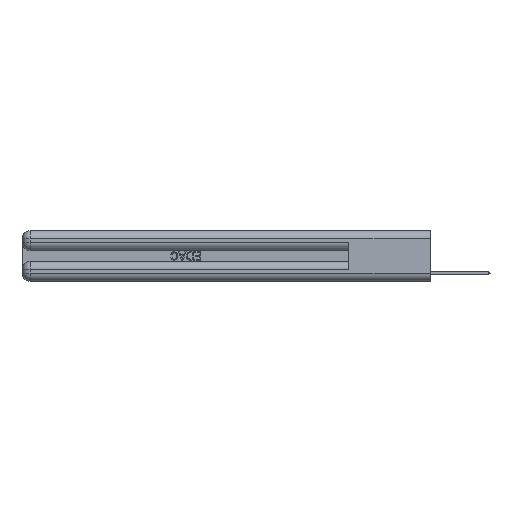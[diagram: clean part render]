
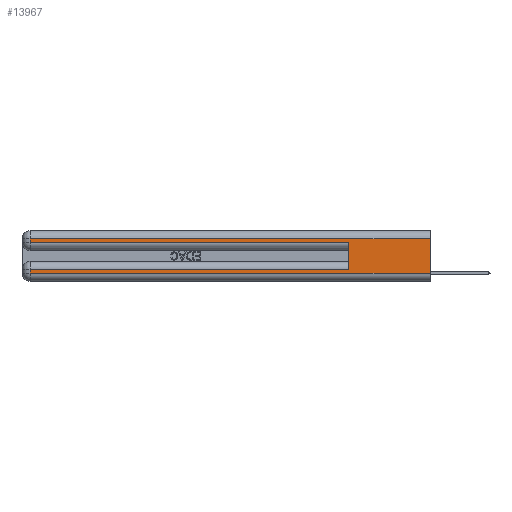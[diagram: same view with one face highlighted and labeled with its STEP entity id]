
A CAD part, left-side view. The second image highlights one B-rep face of the part: STEP entity #13967.
In plain terms, the highlighted planar face has unit normal (-1, 0, 0).
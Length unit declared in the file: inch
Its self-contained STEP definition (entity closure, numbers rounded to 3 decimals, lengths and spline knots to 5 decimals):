
#890 = CARTESIAN_POINT ( 'NONE',  ( 0., 0., 0.37 ) ) ;
#1007 = ORIENTED_EDGE ( 'NONE', *, *, #17822, .T. ) ;
#1080 = ORIENTED_EDGE ( 'NONE', *, *, #3399, .T. ) ;
#1445 = FACE_OUTER_BOUND ( 'NONE', #27630, .T. ) ;
#1595 = LINE ( 'NONE', #23481, #8854 ) ;
#1838 = CARTESIAN_POINT ( 'NONE',  ( 0., 0., 0.06 ) ) ;
#2013 = EDGE_CURVE ( 'NONE', #3633, #29395, #31485, .T. ) ;
#2047 = EDGE_CURVE ( 'NONE', #18196, #31712, #23404, .T. ) ;
#3399 = EDGE_CURVE ( 'NONE', #27878, #25959, #17396, .T. ) ;
#3633 = VERTEX_POINT ( 'NONE', #32773 ) ;
#3682 = VERTEX_POINT ( 'NONE', #33126 ) ;
#4506 = DIRECTION ( 'NONE',  ( 0., 0., -1. ) ) ;
#5807 = CARTESIAN_POINT ( 'NONE',  ( 0., 0., 0.06 ) ) ;
#6829 = ORIENTED_EDGE ( 'NONE', *, *, #7510, .T. ) ;
#7037 = CARTESIAN_POINT ( 'NONE',  ( 0., 2.94, 0.37 ) ) ;
#7241 = VECTOR ( 'NONE', #11696, 39.37008 ) ;
#7389 = CARTESIAN_POINT ( 'NONE',  ( 0., 2.94, 0.37 ) ) ;
#7510 = EDGE_CURVE ( 'NONE', #25959, #31712, #22230, .T. ) ;
#7766 = VECTOR ( 'NONE', #25082, 39.37008 ) ;
#7897 = VECTOR ( 'NONE', #12992, 39.37008 ) ;
#8139 = PLANE ( 'NONE',  #13163 ) ;
#8854 = VECTOR ( 'NONE', #9819, 39.37008 ) ;
#9819 = DIRECTION ( 'NONE',  ( 0., 1., 0. ) ) ;
#11452 = VECTOR ( 'NONE', #25824, 39.37008 ) ;
#11586 = DIRECTION ( 'NONE',  ( 0., 1., 0. ) ) ;
#11696 = DIRECTION ( 'NONE',  ( 0., 0., -1. ) ) ;
#11863 = EDGE_CURVE ( 'NONE', #18196, #24953, #27498, .T. ) ;
#12992 = DIRECTION ( 'NONE',  ( 0., -1., 0. ) ) ;
#13163 = AXIS2_PLACEMENT_3D ( 'NONE', #21433, #29527, #24419 ) ;
#13292 = EDGE_CURVE ( 'NONE', #3682, #29395, #31290, .T. ) ;
#13654 = CARTESIAN_POINT ( 'NONE',  ( 0., 0., 0.31 ) ) ;
#13967 = ADVANCED_FACE ( 'NONE', ( #1445 ), #8139, .F. ) ;
#14440 = VECTOR ( 'NONE', #27520, 39.37008 ) ;
#15915 = CARTESIAN_POINT ( 'NONE',  ( 0., 0., 0.285 ) ) ;
#17396 = LINE ( 'NONE', #7037, #11452 ) ;
#17822 = EDGE_CURVE ( 'NONE', #3633, #27878, #1595, .T. ) ;
#18196 = VERTEX_POINT ( 'NONE', #13654 ) ;
#19053 = CARTESIAN_POINT ( 'NONE',  ( 0., 0.6, 0.145 ) ) ;
#19664 = CARTESIAN_POINT ( 'NONE',  ( 0., 0., 0.31 ) ) ;
#20230 = VECTOR ( 'NONE', #11586, 39.37008 ) ;
#21433 = CARTESIAN_POINT ( 'NONE',  ( 0., 0., 0.37 ) ) ;
#22230 = LINE ( 'NONE', #5807, #7766 ) ;
#22785 = CARTESIAN_POINT ( 'NONE',  ( 0., 2.94, 0.06 ) ) ;
#23404 = LINE ( 'NONE', #890, #7241 ) ;
#23481 = CARTESIAN_POINT ( 'NONE',  ( 0., 0., 0.085 ) ) ;
#23975 = LINE ( 'NONE', #7389, #26538 ) ;
#24419 = DIRECTION ( 'NONE',  ( 0., 0., -1. ) ) ;
#24537 = CARTESIAN_POINT ( 'NONE',  ( 0., 0.6, 0.285 ) ) ;
#24571 = CARTESIAN_POINT ( 'NONE',  ( 0., 2.94, 0.085 ) ) ;
#24953 = VERTEX_POINT ( 'NONE', #30999 ) ;
#24978 = ORIENTED_EDGE ( 'NONE', *, *, #2013, .F. ) ;
#25082 = DIRECTION ( 'NONE',  ( 0., -1., 0. ) ) ;
#25824 = DIRECTION ( 'NONE',  ( 0., 0., -1. ) ) ;
#25959 = VERTEX_POINT ( 'NONE', #22785 ) ;
#26174 = ORIENTED_EDGE ( 'NONE', *, *, #13292, .T. ) ;
#26538 = VECTOR ( 'NONE', #4506, 39.37008 ) ;
#27037 = ORIENTED_EDGE ( 'NONE', *, *, #11863, .T. ) ;
#27457 = ORIENTED_EDGE ( 'NONE', *, *, #2047, .F. ) ;
#27498 = LINE ( 'NONE', #19664, #20230 ) ;
#27520 = DIRECTION ( 'NONE',  ( 0., 0., 1. ) ) ;
#27630 = EDGE_LOOP ( 'NONE', ( #27457, #27037, #33815, #26174, #24978, #1007, #1080, #6829 ) ) ;
#27878 = VERTEX_POINT ( 'NONE', #24571 ) ;
#29395 = VERTEX_POINT ( 'NONE', #24537 ) ;
#29527 = DIRECTION ( 'NONE',  ( 1., 0., 0. ) ) ;
#30999 = CARTESIAN_POINT ( 'NONE',  ( 0., 2.94, 0.31 ) ) ;
#31290 = LINE ( 'NONE', #15915, #7897 ) ;
#31485 = LINE ( 'NONE', #19053, #14440 ) ;
#31712 = VERTEX_POINT ( 'NONE', #1838 ) ;
#32246 = EDGE_CURVE ( 'NONE', #24953, #3682, #23975, .T. ) ;
#32773 = CARTESIAN_POINT ( 'NONE',  ( 0., 0.6, 0.085 ) ) ;
#33126 = CARTESIAN_POINT ( 'NONE',  ( 0., 2.94, 0.285 ) ) ;
#33815 = ORIENTED_EDGE ( 'NONE', *, *, #32246, .T. ) ;
